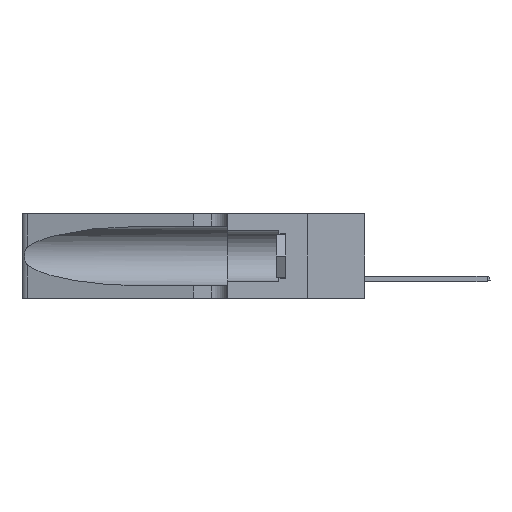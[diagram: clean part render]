
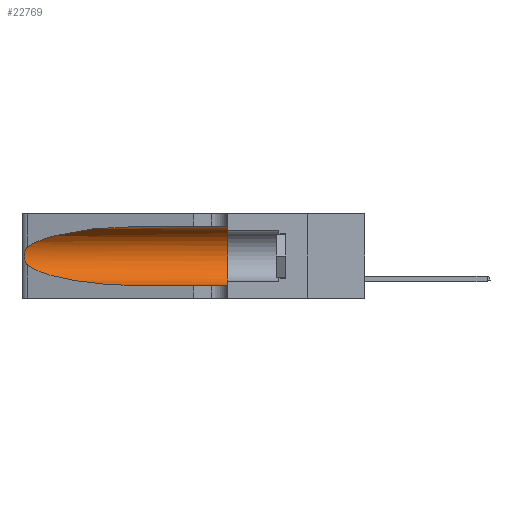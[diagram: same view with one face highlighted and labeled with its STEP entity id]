
A CAD part, left-side view. The second image highlights one B-rep face of the part: STEP entity #22769.
In plain terms, the highlighted cylindrical face has radius 3.308 mm (diameter 6.617 mm), a partial arc.
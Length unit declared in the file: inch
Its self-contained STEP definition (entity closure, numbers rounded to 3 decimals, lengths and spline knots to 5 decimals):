
#8 = CARTESIAN_POINT ( 'NONE',  ( 0.25856, 1.23593, 0.16098 ) ) ;
#189 = EDGE_CURVE ( 'NONE', #4858, #17314, #3486, .T. ) ;
#971 = ORIENTED_EDGE ( 'NONE', *, *, #189, .F. ) ;
#1064 = ORIENTED_EDGE ( 'NONE', *, *, #10167, .T. ) ;
#2306 =( BOUNDED_CURVE ( )  B_SPLINE_CURVE ( 3, ( #14561, #8039, #6188, #23247 ),
 .UNSPECIFIED., .F., .F. ) 
 B_SPLINE_CURVE_WITH_KNOTS ( ( 4, 4 ),
 ( 1.5708, 2.84003 ),
 .UNSPECIFIED. ) 
 CURVE ( )  GEOMETRIC_REPRESENTATION_ITEM ( )  RATIONAL_B_SPLINE_CURVE ( ( 1., 0.87, 0.87, 1. ) ) 
 REPRESENTATION_ITEM ( '' )  );
#2447 = CARTESIAN_POINT ( 'NONE',  ( 0.18966, 0.96281, 0.05475 ) ) ;
#2795 = ORIENTED_EDGE ( 'NONE', *, *, #21663, .T. ) ;
#2805 = CARTESIAN_POINT ( 'NONE',  ( 0.1305, 0.72297, 0.05475 ) ) ;
#3139 = B_SPLINE_CURVE_WITH_KNOTS ( 'NONE', 3,
 ( #21317, #27496, #10711, #23569, #8285, #25556, #10804, #12759, #25644, #8, #14897, #25355, #17026, #27397 ),
 .UNSPECIFIED., .F., .F.,
 ( 4, 2, 2, 2, 2, 2, 4 ),
 ( 0., 0.00027, 0.00053, 0.00107, 0.0016, 0.00187, 0.00214 ),
 .UNSPECIFIED. ) ;
#3486 = LINE ( 'NONE', #12976, #5489 ) ;
#3863 = LINE ( 'NONE', #6379, #9188 ) ;
#3870 = ORIENTED_EDGE ( 'NONE', *, *, #5112, .T. ) ;
#4858 = VERTEX_POINT ( 'NONE', #7261 ) ;
#5112 = EDGE_CURVE ( 'NONE', #9008, #6167, #3863, .T. ) ;
#5443 = CARTESIAN_POINT ( 'NONE',  ( 0.25487, 1.22718, 0.14631 ) ) ;
#5489 = VECTOR ( 'NONE', #23615, 39.37008 ) ;
#5872 = AXIS2_PLACEMENT_3D ( 'NONE', #18843, #19966, #27312 ) ;
#6167 = VERTEX_POINT ( 'NONE', #20954 ) ;
#6188 = CARTESIAN_POINT ( 'NONE',  ( 0.2373, 1.15595, 0.28018 ) ) ;
#6363 = FACE_OUTER_BOUND ( 'NONE', #17344, .T. ) ;
#6379 = CARTESIAN_POINT ( 'NONE',  ( 0.1305, 1.61858, 0.05475 ) ) ;
#6915 = VERTEX_POINT ( 'NONE', #18124 ) ;
#7261 = CARTESIAN_POINT ( 'NONE',  ( 0.1305, 0.72297, 0.31525 ) ) ;
#8039 = CARTESIAN_POINT ( 'NONE',  ( 0.18966, 0.96281, 0.31525 ) ) ;
#8285 = CARTESIAN_POINT ( 'NONE',  ( 0.25854, 1.2359, 0.20912 ) ) ;
#9008 = VERTEX_POINT ( 'NONE', #18144 ) ;
#9188 = VECTOR ( 'NONE', #23526, 39.37008 ) ;
#9326 = CIRCLE ( 'NONE', #9430, 0.13025 ) ;
#9430 = AXIS2_PLACEMENT_3D ( 'NONE', #25961, #17437, #15304 ) ;
#9505 = ORIENTED_EDGE ( 'NONE', *, *, #23276, .T. ) ;
#9651 = CARTESIAN_POINT ( 'NONE',  ( 0.1305, 0.35, 0.31525 ) ) ;
#10167 = EDGE_CURVE ( 'NONE', #4858, #6915, #2306, .T. ) ;
#10711 = CARTESIAN_POINT ( 'NONE',  ( 0.25639, 1.23184, 0.21858 ) ) ;
#10804 = CARTESIAN_POINT ( 'NONE',  ( 0.26075, 1.23896, 0.19203 ) ) ;
#12759 = CARTESIAN_POINT ( 'NONE',  ( 0.26075, 1.23896, 0.178 ) ) ;
#12976 = CARTESIAN_POINT ( 'NONE',  ( 0.1305, 1.61858, 0.31525 ) ) ;
#13259 = ORIENTED_EDGE ( 'NONE', *, *, #25107, .F. ) ;
#13835 = VERTEX_POINT ( 'NONE', #5443 ) ;
#14561 = CARTESIAN_POINT ( 'NONE',  ( 0.1305, 0.72297, 0.31525 ) ) ;
#14897 = CARTESIAN_POINT ( 'NONE',  ( 0.25789, 1.23486, 0.15765 ) ) ;
#15304 = DIRECTION ( 'NONE',  ( 0., 0., 1. ) ) ;
#17026 = CARTESIAN_POINT ( 'NONE',  ( 0.25555, 1.22993, 0.14849 ) ) ;
#17314 = VERTEX_POINT ( 'NONE', #9651 ) ;
#17344 = EDGE_LOOP ( 'NONE', ( #1064, #2795, #9505, #3870, #13259, #971 ) ) ;
#17437 = DIRECTION ( 'NONE',  ( 0., 1., 0. ) ) ;
#17703 = CARTESIAN_POINT ( 'NONE',  ( 0.25487, 1.22718, 0.14631 ) ) ;
#18124 = CARTESIAN_POINT ( 'NONE',  ( 0.25487, 1.22718, 0.22369 ) ) ;
#18144 = CARTESIAN_POINT ( 'NONE',  ( 0.1305, 0.72297, 0.05475 ) ) ;
#18843 = CARTESIAN_POINT ( 'NONE',  ( 0.1305, 1.61858, 0.185 ) ) ;
#18864 =( BOUNDED_CURVE ( )  B_SPLINE_CURVE ( 3, ( #17703, #21815, #2447, #2805 ),
 .UNSPECIFIED., .F., .T. ) 
 B_SPLINE_CURVE_WITH_KNOTS ( ( 4, 4 ),
 ( 3.44316, 4.71239 ),
 .UNSPECIFIED. ) 
 CURVE ( )  GEOMETRIC_REPRESENTATION_ITEM ( )  RATIONAL_B_SPLINE_CURVE ( ( 1., 0.87, 0.87, 1. ) ) 
 REPRESENTATION_ITEM ( '' )  );
#19691 = CYLINDRICAL_SURFACE ( 'NONE', #5872, 0.13025 ) ;
#19966 = DIRECTION ( 'NONE',  ( 0., -1., 0. ) ) ;
#20954 = CARTESIAN_POINT ( 'NONE',  ( 0.1305, 0.35, 0.05475 ) ) ;
#21317 = CARTESIAN_POINT ( 'NONE',  ( 0.25487, 1.22718, 0.22369 ) ) ;
#21663 = EDGE_CURVE ( 'NONE', #6915, #13835, #3139, .T. ) ;
#21815 = CARTESIAN_POINT ( 'NONE',  ( 0.2373, 1.15595, 0.08982 ) ) ;
#22769 = ADVANCED_FACE ( 'NONE', ( #6363 ), #19691, .F. ) ;
#23247 = CARTESIAN_POINT ( 'NONE',  ( 0.25487, 1.22718, 0.22369 ) ) ;
#23276 = EDGE_CURVE ( 'NONE', #13835, #9008, #18864, .T. ) ;
#23526 = DIRECTION ( 'NONE',  ( 0., -1., 0. ) ) ;
#23569 = CARTESIAN_POINT ( 'NONE',  ( 0.25787, 1.23484, 0.2124 ) ) ;
#23615 = DIRECTION ( 'NONE',  ( 0., -1., 0. ) ) ;
#25107 = EDGE_CURVE ( 'NONE', #17314, #6167, #9326, .T. ) ;
#25355 = CARTESIAN_POINT ( 'NONE',  ( 0.25639, 1.23186, 0.15144 ) ) ;
#25556 = CARTESIAN_POINT ( 'NONE',  ( 0.26018, 1.23835, 0.19895 ) ) ;
#25644 = CARTESIAN_POINT ( 'NONE',  ( 0.26017, 1.23833, 0.17102 ) ) ;
#25961 = CARTESIAN_POINT ( 'NONE',  ( 0.1305, 0.35, 0.185 ) ) ;
#27312 = DIRECTION ( 'NONE',  ( 0., 0., -1. ) ) ;
#27397 = CARTESIAN_POINT ( 'NONE',  ( 0.25487, 1.22718, 0.14631 ) ) ;
#27496 = CARTESIAN_POINT ( 'NONE',  ( 0.25555, 1.22994, 0.2215 ) ) ;
